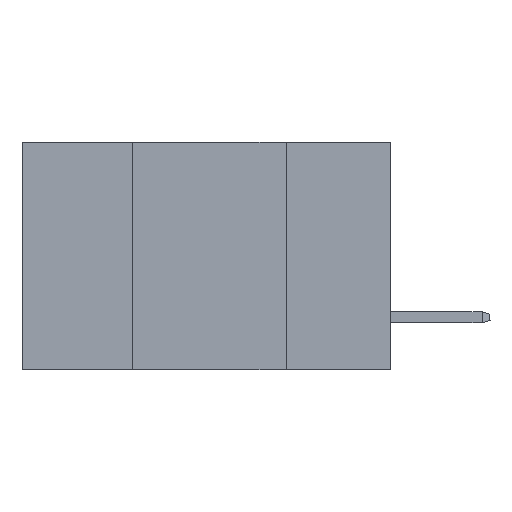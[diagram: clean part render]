
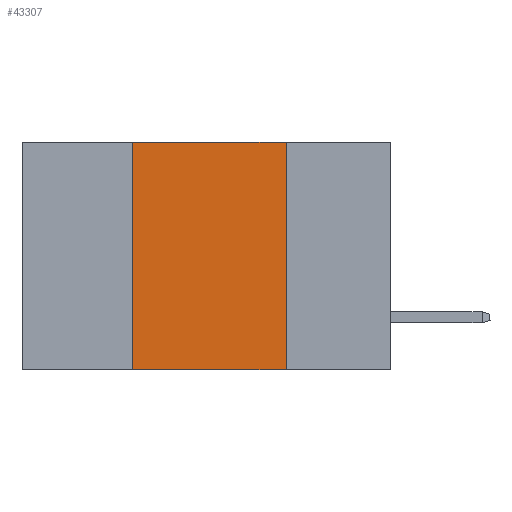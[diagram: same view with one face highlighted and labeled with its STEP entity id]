
A CAD part, left-side view. The second image highlights one B-rep face of the part: STEP entity #43307.
In plain terms, the highlighted planar face has unit normal (-1, 0, 0).
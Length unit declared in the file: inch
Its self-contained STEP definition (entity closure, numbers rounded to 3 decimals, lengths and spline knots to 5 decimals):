
#262 = LINE ( 'NONE', #35322, #30538 ) ;
#2741 = VECTOR ( 'NONE', #3341, 39.37008 ) ;
#3341 = DIRECTION ( 'NONE',  ( 0., 0., 1. ) ) ;
#4141 = CARTESIAN_POINT ( 'NONE',  ( 0., 0.6, 0. ) ) ;
#7816 = ORIENTED_EDGE ( 'NONE', *, *, #23635, .F. ) ;
#8013 = DIRECTION ( 'NONE',  ( 0., -1., 0. ) ) ;
#8726 = DIRECTION ( 'NONE',  ( 0., -1., 0. ) ) ;
#9731 = EDGE_CURVE ( 'NONE', #11678, #24309, #262, .T. ) ;
#11678 = VERTEX_POINT ( 'NONE', #43196 ) ;
#13110 = VECTOR ( 'NONE', #47400, 39.37008 ) ;
#14394 = ORIENTED_EDGE ( 'NONE', *, *, #9731, .T. ) ;
#15805 = ORIENTED_EDGE ( 'NONE', *, *, #23047, .F. ) ;
#16506 = AXIS2_PLACEMENT_3D ( 'NONE', #4141, #46302, #38817 ) ;
#21226 = VECTOR ( 'NONE', #8013, 39.37008 ) ;
#23047 = EDGE_CURVE ( 'NONE', #27609, #27762, #40880, .T. ) ;
#23544 = CARTESIAN_POINT ( 'NONE',  ( 0., 0.42, 0. ) ) ;
#23635 = EDGE_CURVE ( 'NONE', #11678, #27609, #48486, .T. ) ;
#24309 = VERTEX_POINT ( 'NONE', #26019 ) ;
#26019 = CARTESIAN_POINT ( 'NONE',  ( 0., 0.17, -0.37 ) ) ;
#27609 = VERTEX_POINT ( 'NONE', #23544 ) ;
#27762 = VERTEX_POINT ( 'NONE', #46971 ) ;
#28359 = EDGE_CURVE ( 'NONE', #27762, #24309, #39301, .T. ) ;
#29901 = FACE_OUTER_BOUND ( 'NONE', #38955, .T. ) ;
#30538 = VECTOR ( 'NONE', #8726, 39.37008 ) ;
#35322 = CARTESIAN_POINT ( 'NONE',  ( 0., 0.6, -0.37 ) ) ;
#37846 = CARTESIAN_POINT ( 'NONE',  ( 0., 0.42, 0. ) ) ;
#38817 = DIRECTION ( 'NONE',  ( 0., 0., -1. ) ) ;
#38955 = EDGE_LOOP ( 'NONE', ( #45295, #15805, #7816, #14394 ) ) ;
#39301 = LINE ( 'NONE', #43918, #13110 ) ;
#40880 = LINE ( 'NONE', #41574, #21226 ) ;
#41574 = CARTESIAN_POINT ( 'NONE',  ( 0., 0.6, 0. ) ) ;
#42474 = PLANE ( 'NONE',  #16506 ) ;
#43196 = CARTESIAN_POINT ( 'NONE',  ( 0., 0.42, -0.37 ) ) ;
#43307 = ADVANCED_FACE ( 'NONE', ( #29901 ), #42474, .F. ) ;
#43918 = CARTESIAN_POINT ( 'NONE',  ( 0., 0.17, 0. ) ) ;
#45295 = ORIENTED_EDGE ( 'NONE', *, *, #28359, .F. ) ;
#46302 = DIRECTION ( 'NONE',  ( 1., 0., 0. ) ) ;
#46971 = CARTESIAN_POINT ( 'NONE',  ( 0., 0.17, 0. ) ) ;
#47400 = DIRECTION ( 'NONE',  ( 0., 0., -1. ) ) ;
#48486 = LINE ( 'NONE', #37846, #2741 ) ;
